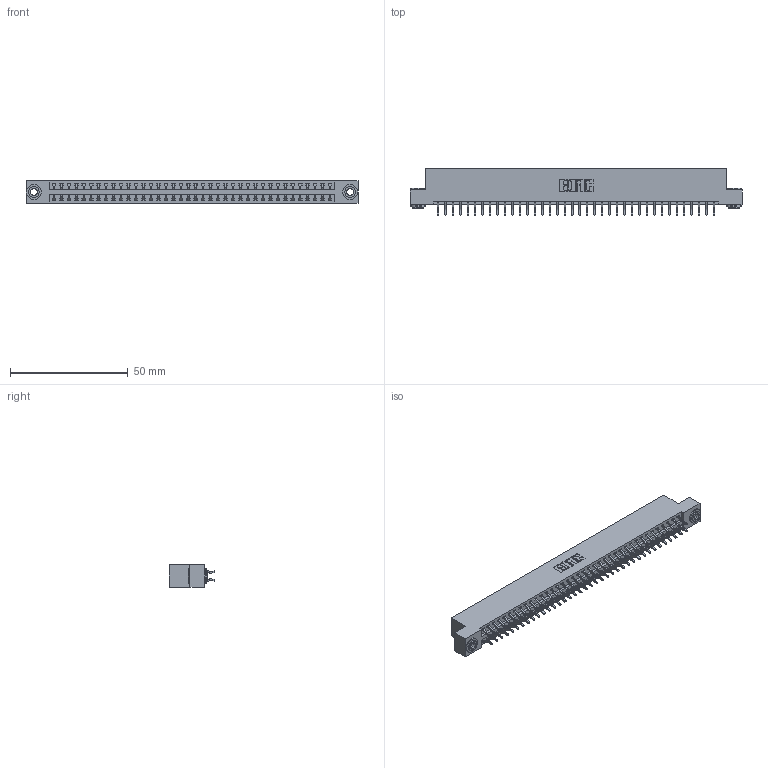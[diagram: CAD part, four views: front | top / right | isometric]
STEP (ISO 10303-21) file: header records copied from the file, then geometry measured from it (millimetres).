
FILE_DESCRIPTION (( 'STEP AP203' ), '1' );
FILE_NAME ('396-076-556-203.STEP', '2019-10-30T21:37:27', ( '' ), ( '' ), 'SwSTEP 2.0', 'SolidWorks 2016', '' );
FILE_SCHEMA (( 'CONFIG_CONTROL_DESIGN' ));
Length unit declared in the file: inch
Products named in the file (4): 396-076-556-203; 346 Part_Flush Mounting Lugs - 0.156 Dia-TH; 345-292-001_556 Tail; 345-250-002_345-250-002-102
Assembly tree (79 placements, depth 2):
  396-076-556-203
    346 Part_Flush Mounting Lugs - 0.156 Dia-TH
    345-292-001_556 Tail  x76
    345-250-002_345-250-002-102  x2
Bounding box: 141.22 x 19.57 x 9.4 mm (x, y, z)
Volume: 13756.4 mm3; surface area: 18989.8 mm2
Topology: 79 solids, 79 shells, 4568 faces, 13553 edges, 8930 vertices
Faces by surface type: plane 3050, cylinder 1510, cone 8
Entity records: 26208 total; most frequent: CARTESIAN_POINT 4315, ORIENTED_EDGE 4230, DIRECTION 3873, EDGE_CURVE 2115, LINE 1799, VECTOR 1799, VERTEX_POINT 1406, AXIS2_PLACEMENT_3D 1037
